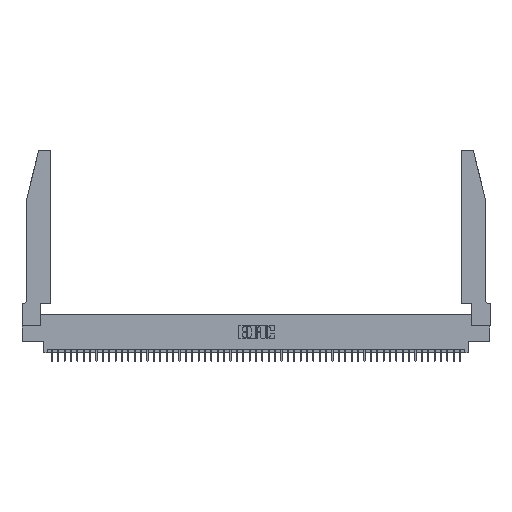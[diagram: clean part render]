
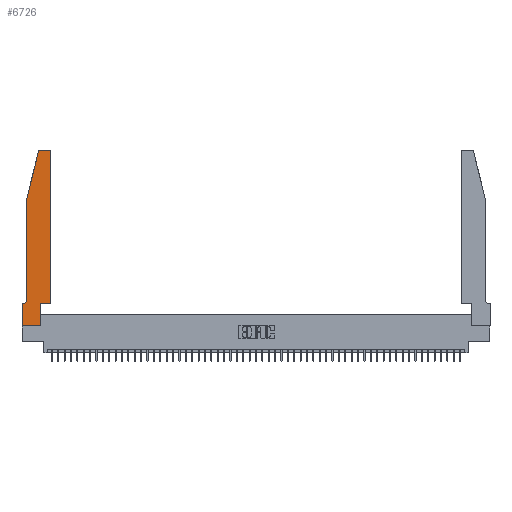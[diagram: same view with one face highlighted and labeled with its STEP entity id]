
A CAD part, top view. The second image highlights one B-rep face of the part: STEP entity #6726.
In plain terms, the highlighted planar face has unit normal (0, 0, 1).
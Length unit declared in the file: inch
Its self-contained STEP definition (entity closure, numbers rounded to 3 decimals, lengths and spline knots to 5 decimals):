
#120 = LINE ( 'NONE', #16421, #39590 ) ;
#158 = DIRECTION ( 'NONE',  ( 1., 0., 0. ) ) ;
#478 = DIRECTION ( 'NONE',  ( 1., 0., 0. ) ) ;
#604 = CARTESIAN_POINT ( 'NONE',  ( 0., 0.35, 0.37 ) ) ;
#728 = EDGE_CURVE ( 'NONE', #11628, #13694, #14811, .T. ) ;
#2886 = VERTEX_POINT ( 'NONE', #29647 ) ;
#3319 = ORIENTED_EDGE ( 'NONE', *, *, #45950, .T. ) ;
#3485 = ORIENTED_EDGE ( 'NONE', *, *, #15709, .T. ) ;
#3758 = CIRCLE ( 'NONE', #24224, 0.07 ) ;
#4239 = DIRECTION ( 'NONE',  ( -1., 0., 0. ) ) ;
#4743 = DIRECTION ( 'NONE',  ( 0., 0., 1. ) ) ;
#5067 = LINE ( 'NONE', #33766, #14963 ) ;
#5840 = CARTESIAN_POINT ( 'NONE',  ( 0.0055, 0.35, 0.37 ) ) ;
#6354 = VERTEX_POINT ( 'NONE', #34622 ) ;
#6726 = ADVANCED_FACE ( 'NONE', ( #49441 ), #45445, .T. ) ;
#8018 = EDGE_CURVE ( 'NONE', #6354, #15029, #120, .T. ) ;
#8730 = DIRECTION ( 'NONE',  ( 1., 0., 0. ) ) ;
#9738 = DIRECTION ( 'NONE',  ( 1., 0., 0. ) ) ;
#9762 = VECTOR ( 'NONE', #158, 39.37008 ) ;
#10664 = ORIENTED_EDGE ( 'NONE', *, *, #26440, .T. ) ;
#11628 = VERTEX_POINT ( 'NONE', #12344 ) ;
#12344 = CARTESIAN_POINT ( 'NONE',  ( 0.4505, 2.72, 0.37 ) ) ;
#12366 = LINE ( 'NONE', #16096, #21913 ) ;
#12439 = LINE ( 'NONE', #21019, #9762 ) ;
#13124 = VERTEX_POINT ( 'NONE', #604 ) ;
#13235 = ORIENTED_EDGE ( 'NONE', *, *, #23717, .T. ) ;
#13694 = VERTEX_POINT ( 'NONE', #23600 ) ;
#14811 = CIRCLE ( 'NONE', #16249, 0.03 ) ;
#14963 = VECTOR ( 'NONE', #46330, 39.37008 ) ;
#15029 = VERTEX_POINT ( 'NONE', #26514 ) ;
#15709 = EDGE_CURVE ( 'NONE', #13694, #35930, #25337, .T. ) ;
#15834 = CARTESIAN_POINT ( 'NONE',  ( 0.284, 2.75, 0.37 ) ) ;
#16096 = CARTESIAN_POINT ( 'NONE',  ( 0.4505, 0.35, 0.37 ) ) ;
#16154 = ORIENTED_EDGE ( 'NONE', *, *, #8018, .T. ) ;
#16249 = AXIS2_PLACEMENT_3D ( 'NONE', #30955, #18048, #9738 ) ;
#16421 = CARTESIAN_POINT ( 'NONE',  ( 0.2865, 0.35, 0.37 ) ) ;
#17070 = ORIENTED_EDGE ( 'NONE', *, *, #728, .T. ) ;
#17510 = LINE ( 'NONE', #41400, #33832 ) ;
#17577 = DIRECTION ( 'NONE',  ( 0., 0., 1. ) ) ;
#18048 = DIRECTION ( 'NONE',  ( 0., 0., 1. ) ) ;
#18052 = ORIENTED_EDGE ( 'NONE', *, *, #38352, .T. ) ;
#18154 = CARTESIAN_POINT ( 'NONE',  ( 0.0755, 0.42, 0.37 ) ) ;
#18670 = VECTOR ( 'NONE', #4239, 39.37008 ) ;
#19906 = VERTEX_POINT ( 'NONE', #34450 ) ;
#20928 = DIRECTION ( 'NONE',  ( -1., 0., 0. ) ) ;
#20971 = CARTESIAN_POINT ( 'NONE',  ( 0.4505, 0.35, 0.37 ) ) ;
#21019 = CARTESIAN_POINT ( 'NONE',  ( 0., 0., 0.37 ) ) ;
#21913 = VECTOR ( 'NONE', #40276, 39.37008 ) ;
#22269 = VECTOR ( 'NONE', #23991, 39.37008 ) ;
#23600 = CARTESIAN_POINT ( 'NONE',  ( 0.4205, 2.75, 0.37 ) ) ;
#23663 = CIRCLE ( 'NONE', #34011, 0.03 ) ;
#23717 = EDGE_CURVE ( 'NONE', #26411, #6354, #12439, .T. ) ;
#23991 = DIRECTION ( 'NONE',  ( 1., 0., 0. ) ) ;
#24224 = AXIS2_PLACEMENT_3D ( 'NONE', #33840, #41845, #20928 ) ;
#25337 = LINE ( 'NONE', #41695, #18670 ) ;
#25771 = AXIS2_PLACEMENT_3D ( 'NONE', #32611, #4743, #8730 ) ;
#25925 = VERTEX_POINT ( 'NONE', #5840 ) ;
#25965 = DIRECTION ( 'NONE',  ( 0., -1., 0. ) ) ;
#26365 = CARTESIAN_POINT ( 'NONE',  ( 0.25487, 2.72718, 0.37 ) ) ;
#26411 = VERTEX_POINT ( 'NONE', #50237 ) ;
#26440 = EDGE_CURVE ( 'NONE', #13124, #26411, #39561, .T. ) ;
#26514 = CARTESIAN_POINT ( 'NONE',  ( 0.2865, 0.35, 0.37 ) ) ;
#27089 = ORIENTED_EDGE ( 'NONE', *, *, #50946, .T. ) ;
#28033 = LINE ( 'NONE', #20971, #22269 ) ;
#28492 = EDGE_CURVE ( 'NONE', #25925, #13124, #5067, .T. ) ;
#29211 = ORIENTED_EDGE ( 'NONE', *, *, #37094, .T. ) ;
#29647 = CARTESIAN_POINT ( 'NONE',  ( 0.0755, 2., 0.37 ) ) ;
#30955 = CARTESIAN_POINT ( 'NONE',  ( 0.4205, 2.72, 0.37 ) ) ;
#32611 = CARTESIAN_POINT ( 'NONE',  ( 0., 0.35, 0.37 ) ) ;
#32829 = DIRECTION ( 'NONE',  ( 0., 1., 0. ) ) ;
#33766 = CARTESIAN_POINT ( 'NONE',  ( 0.0755, 0.35, 0.37 ) ) ;
#33832 = VECTOR ( 'NONE', #41653, 39.37008 ) ;
#33840 = CARTESIAN_POINT ( 'NONE',  ( 0.0055, 0.42, 0.37 ) ) ;
#33872 = EDGE_CURVE ( 'NONE', #46302, #2886, #17510, .T. ) ;
#34011 = AXIS2_PLACEMENT_3D ( 'NONE', #37215, #17577, #478 ) ;
#34043 = CARTESIAN_POINT ( 'NONE',  ( 0.0755, 2., 0.37 ) ) ;
#34450 = CARTESIAN_POINT ( 'NONE',  ( 0.4505, 0.35, 0.37 ) ) ;
#34622 = CARTESIAN_POINT ( 'NONE',  ( 0.2865, 0., 0.37 ) ) ;
#35930 = VERTEX_POINT ( 'NONE', #15834 ) ;
#36822 = EDGE_LOOP ( 'NONE', ( #3485, #18052, #46470, #3319, #27089, #49501, #10664, #13235, #16154, #48704, #29211, #17070 ) ) ;
#37094 = EDGE_CURVE ( 'NONE', #19906, #11628, #12366, .T. ) ;
#37215 = CARTESIAN_POINT ( 'NONE',  ( 0.284, 2.72, 0.37 ) ) ;
#38329 = LINE ( 'NONE', #34043, #41246 ) ;
#38352 = EDGE_CURVE ( 'NONE', #35930, #46302, #23663, .T. ) ;
#39561 = LINE ( 'NONE', #51313, #40076 ) ;
#39590 = VECTOR ( 'NONE', #32829, 39.37008 ) ;
#40076 = VECTOR ( 'NONE', #43278, 39.37008 ) ;
#40276 = DIRECTION ( 'NONE',  ( 0., 1., 0. ) ) ;
#41246 = VECTOR ( 'NONE', #25965, 39.37008 ) ;
#41400 = CARTESIAN_POINT ( 'NONE',  ( 0.0755, 2., 0.37 ) ) ;
#41653 = DIRECTION ( 'NONE',  ( -0.239, -0.971, 0. ) ) ;
#41695 = CARTESIAN_POINT ( 'NONE',  ( 0.2605, 2.75, 0.37 ) ) ;
#41845 = DIRECTION ( 'NONE',  ( 0., 0., -1. ) ) ;
#43278 = DIRECTION ( 'NONE',  ( 0., -1., 0. ) ) ;
#45445 = PLANE ( 'NONE',  #25771 ) ;
#45950 = EDGE_CURVE ( 'NONE', #2886, #48397, #38329, .T. ) ;
#46302 = VERTEX_POINT ( 'NONE', #26365 ) ;
#46330 = DIRECTION ( 'NONE',  ( -1., 0., 0. ) ) ;
#46470 = ORIENTED_EDGE ( 'NONE', *, *, #33872, .T. ) ;
#47174 = EDGE_CURVE ( 'NONE', #15029, #19906, #28033, .T. ) ;
#48397 = VERTEX_POINT ( 'NONE', #18154 ) ;
#48704 = ORIENTED_EDGE ( 'NONE', *, *, #47174, .T. ) ;
#49441 = FACE_OUTER_BOUND ( 'NONE', #36822, .T. ) ;
#49501 = ORIENTED_EDGE ( 'NONE', *, *, #28492, .T. ) ;
#50237 = CARTESIAN_POINT ( 'NONE',  ( 0., 0., 0.37 ) ) ;
#50946 = EDGE_CURVE ( 'NONE', #48397, #25925, #3758, .T. ) ;
#51313 = CARTESIAN_POINT ( 'NONE',  ( 0., 0., 0.37 ) ) ;
